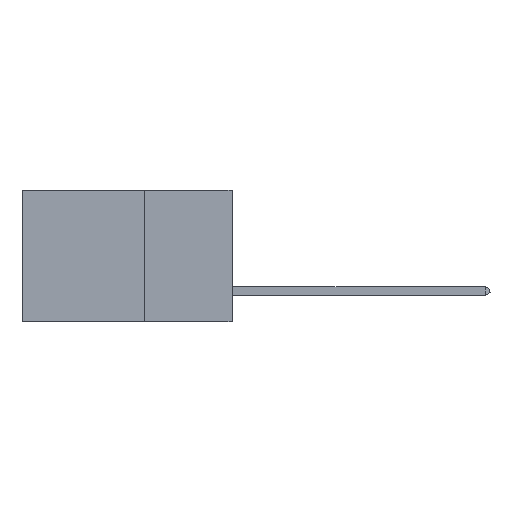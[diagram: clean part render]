
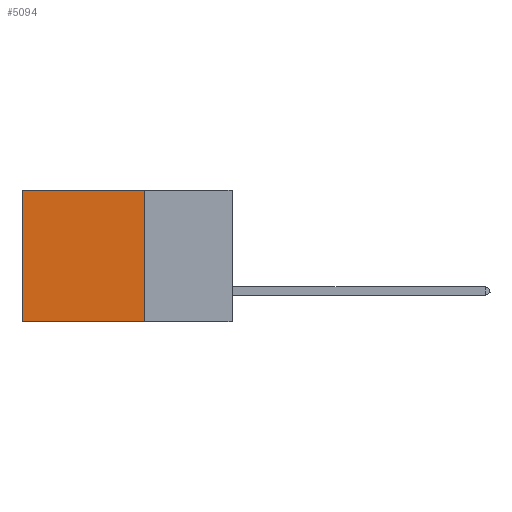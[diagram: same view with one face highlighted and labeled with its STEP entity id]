
A CAD part, left-side view. The second image highlights one B-rep face of the part: STEP entity #5094.
In plain terms, the highlighted planar face has unit normal (-1, 0, 0).
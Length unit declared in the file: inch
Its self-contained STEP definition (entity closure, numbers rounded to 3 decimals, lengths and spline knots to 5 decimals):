
#531 = DIRECTION ( 'NONE',  ( 0., 1., 0. ) ) ;
#1515 = VERTEX_POINT ( 'NONE', #6350 ) ;
#1804 = ORIENTED_EDGE ( 'NONE', *, *, #15547, .F. ) ;
#1821 = LINE ( 'NONE', #15491, #12364 ) ;
#2464 = PLANE ( 'NONE',  #14305 ) ;
#3896 = FACE_OUTER_BOUND ( 'NONE', #8829, .T. ) ;
#3931 = DIRECTION ( 'NONE',  ( 1., 0., 0. ) ) ;
#4528 = LINE ( 'NONE', #10914, #10964 ) ;
#5094 = ADVANCED_FACE ( 'NONE', ( #3896 ), #2464, .F. ) ;
#5166 = DIRECTION ( 'NONE',  ( 0., 0., -1. ) ) ;
#5838 = CARTESIAN_POINT ( 'NONE',  ( 0.2875, 0.25, -0.375 ) ) ;
#6350 = CARTESIAN_POINT ( 'NONE',  ( 0.2875, 0.25, 0. ) ) ;
#6599 = VECTOR ( 'NONE', #11553, 39.37008 ) ;
#6652 = CARTESIAN_POINT ( 'NONE',  ( 0.2875, 0.25, -0.375 ) ) ;
#8244 = CARTESIAN_POINT ( 'NONE',  ( 0.2875, 0.6, 0. ) ) ;
#8631 = ORIENTED_EDGE ( 'NONE', *, *, #10543, .T. ) ;
#8829 = EDGE_LOOP ( 'NONE', ( #10959, #1804, #14544, #8631 ) ) ;
#9064 = EDGE_CURVE ( 'NONE', #11388, #9756, #1821, .T. ) ;
#9756 = VERTEX_POINT ( 'NONE', #12587 ) ;
#10543 = EDGE_CURVE ( 'NONE', #1515, #11388, #4528, .T. ) ;
#10914 = CARTESIAN_POINT ( 'NONE',  ( 0.2875, 0.25, 0. ) ) ;
#10958 = CARTESIAN_POINT ( 'NONE',  ( 0.2875, 0.25, -0.375 ) ) ;
#10959 = ORIENTED_EDGE ( 'NONE', *, *, #9064, .T. ) ;
#10964 = VECTOR ( 'NONE', #531, 39.37008 ) ;
#11097 = DIRECTION ( 'NONE',  ( 0., 0., -1. ) ) ;
#11388 = VERTEX_POINT ( 'NONE', #8244 ) ;
#11553 = DIRECTION ( 'NONE',  ( 0., 1., 0. ) ) ;
#11751 = VECTOR ( 'NONE', #13501, 39.37008 ) ;
#12209 = EDGE_CURVE ( 'NONE', #1515, #18684, #14905, .T. ) ;
#12364 = VECTOR ( 'NONE', #11097, 39.37008 ) ;
#12587 = CARTESIAN_POINT ( 'NONE',  ( 0.2875, 0.6, -0.375 ) ) ;
#13501 = DIRECTION ( 'NONE',  ( 0., 0., -1. ) ) ;
#14305 = AXIS2_PLACEMENT_3D ( 'NONE', #6652, #3931, #5166 ) ;
#14544 = ORIENTED_EDGE ( 'NONE', *, *, #12209, .F. ) ;
#14767 = CARTESIAN_POINT ( 'NONE',  ( 0.2875, 0.25, -0.375 ) ) ;
#14905 = LINE ( 'NONE', #14767, #11751 ) ;
#15491 = CARTESIAN_POINT ( 'NONE',  ( 0.2875, 0.6, -0.375 ) ) ;
#15547 = EDGE_CURVE ( 'NONE', #18684, #9756, #17135, .T. ) ;
#17135 = LINE ( 'NONE', #5838, #6599 ) ;
#18684 = VERTEX_POINT ( 'NONE', #10958 ) ;
